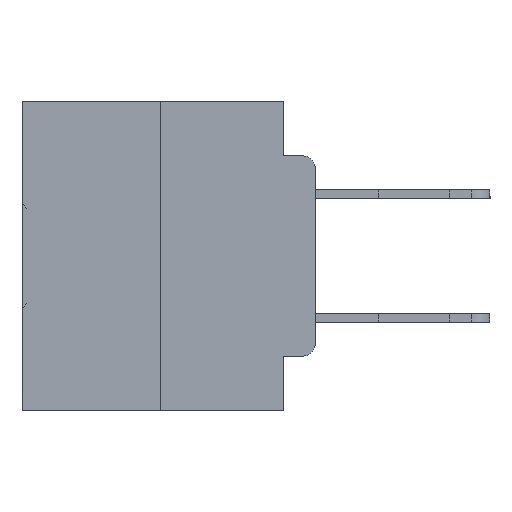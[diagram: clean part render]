
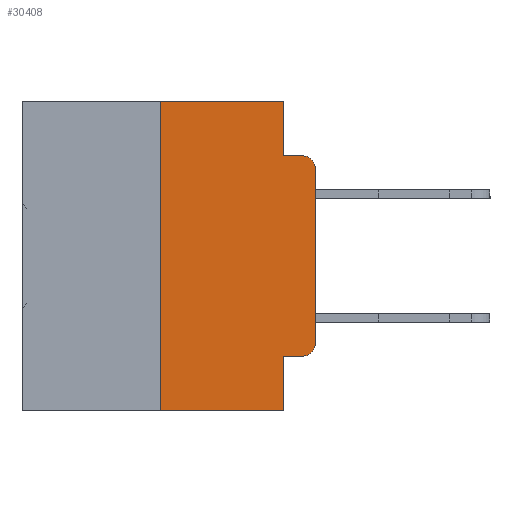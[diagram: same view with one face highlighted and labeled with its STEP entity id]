
A CAD part, left-side view. The second image highlights one B-rep face of the part: STEP entity #30408.
In plain terms, the highlighted planar face has unit normal (-1, 0, 0).
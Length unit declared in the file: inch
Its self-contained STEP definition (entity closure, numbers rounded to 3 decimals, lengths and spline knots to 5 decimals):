
#230 = DIRECTION ( 'NONE',  ( 0., 0., 1. ) ) ;
#309 = CARTESIAN_POINT ( 'NONE',  ( 0., 0.02, -0.4115 ) ) ;
#893 = AXIS2_PLACEMENT_3D ( 'NONE', #1442, #27420, #12068 ) ;
#911 = ORIENTED_EDGE ( 'NONE', *, *, #17243, .F. ) ;
#1036 = VECTOR ( 'NONE', #23882, 39.37008 ) ;
#1442 = CARTESIAN_POINT ( 'NONE',  ( 0., 0.473, 0. ) ) ;
#1462 = DIRECTION ( 'NONE',  ( -1., 0., 0. ) ) ;
#1540 = LINE ( 'NONE', #7301, #21604 ) ;
#2047 = AXIS2_PLACEMENT_3D ( 'NONE', #17199, #1462, #19800 ) ;
#2131 = VECTOR ( 'NONE', #27303, 39.37008 ) ;
#2607 = CARTESIAN_POINT ( 'NONE',  ( 0., 0.051, -0.4115 ) ) ;
#3167 = CARTESIAN_POINT ( 'NONE',  ( 0., 0.051, 0. ) ) ;
#3987 = DIRECTION ( 'NONE',  ( -1., 0., 0. ) ) ;
#4912 = EDGE_CURVE ( 'NONE', #25032, #22070, #17927, .T. ) ;
#5413 = LINE ( 'NONE', #2607, #19292 ) ;
#5738 = DIRECTION ( 'NONE',  ( 0., -1., 0. ) ) ;
#6139 = AXIS2_PLACEMENT_3D ( 'NONE', #19637, #3987, #22230 ) ;
#6345 = ORIENTED_EDGE ( 'NONE', *, *, #9194, .F. ) ;
#6702 = CARTESIAN_POINT ( 'NONE',  ( 0., 0.473, 0. ) ) ;
#6966 = LINE ( 'NONE', #25739, #15532 ) ;
#7089 = EDGE_CURVE ( 'NONE', #31402, #33297, #17375, .T. ) ;
#7301 = CARTESIAN_POINT ( 'NONE',  ( 0., 0.473, -0.5 ) ) ;
#7318 = CARTESIAN_POINT ( 'NONE',  ( 0., 0.051, 0. ) ) ;
#7378 = ORIENTED_EDGE ( 'NONE', *, *, #21119, .T. ) ;
#7640 = FACE_OUTER_BOUND ( 'NONE', #31909, .T. ) ;
#7711 = DIRECTION ( 'NONE',  ( 0., 0., 1. ) ) ;
#7778 = VERTEX_POINT ( 'NONE', #29662 ) ;
#9156 = VERTEX_POINT ( 'NONE', #15133 ) ;
#9183 = LINE ( 'NONE', #6702, #2131 ) ;
#9194 = EDGE_CURVE ( 'NONE', #7778, #32922, #9557, .T. ) ;
#9280 = ORIENTED_EDGE ( 'NONE', *, *, #4912, .F. ) ;
#9343 = EDGE_CURVE ( 'NONE', #25032, #31402, #5413, .T. ) ;
#9557 = LINE ( 'NONE', #23004, #15660 ) ;
#10035 = VECTOR ( 'NONE', #230, 39.37008 ) ;
#11731 = EDGE_CURVE ( 'NONE', #33297, #32806, #6966, .T. ) ;
#12068 = DIRECTION ( 'NONE',  ( 0., 0., -1. ) ) ;
#12513 = DIRECTION ( 'NONE',  ( 0., -1., 0. ) ) ;
#13423 = CARTESIAN_POINT ( 'NONE',  ( 0., 0.25, 0. ) ) ;
#14202 = CARTESIAN_POINT ( 'NONE',  ( 0., 0.02, -0.0885 ) ) ;
#14265 = LINE ( 'NONE', #3167, #1036 ) ;
#15133 = CARTESIAN_POINT ( 'NONE',  ( 0., 0.25, 0. ) ) ;
#15532 = VECTOR ( 'NONE', #7711, 39.37008 ) ;
#15660 = VECTOR ( 'NONE', #12513, 39.37008 ) ;
#16231 = CIRCLE ( 'NONE', #2047, 0.02 ) ;
#16683 = CARTESIAN_POINT ( 'NONE',  ( 0., 0.25, -0.5 ) ) ;
#17199 = CARTESIAN_POINT ( 'NONE',  ( 0., 0.02, -0.1085 ) ) ;
#17243 = EDGE_CURVE ( 'NONE', #9156, #23777, #9183, .T. ) ;
#17375 = CIRCLE ( 'NONE', #6139, 0.02 ) ;
#17927 = LINE ( 'NONE', #21235, #24719 ) ;
#19190 = DIRECTION ( 'NONE',  ( 0., 0., -1. ) ) ;
#19292 = VECTOR ( 'NONE', #5738, 39.37008 ) ;
#19384 = EDGE_CURVE ( 'NONE', #26133, #22070, #1540, .T. ) ;
#19637 = CARTESIAN_POINT ( 'NONE',  ( 0., 0.02, -0.3915 ) ) ;
#19774 = PLANE ( 'NONE',  #893 ) ;
#19800 = DIRECTION ( 'NONE',  ( 0., 0., -1. ) ) ;
#21119 = EDGE_CURVE ( 'NONE', #32806, #32922, #16231, .T. ) ;
#21235 = CARTESIAN_POINT ( 'NONE',  ( 0., 0.051, 0. ) ) ;
#21604 = VECTOR ( 'NONE', #25354, 39.37008 ) ;
#21758 = ORIENTED_EDGE ( 'NONE', *, *, #25485, .F. ) ;
#22036 = CARTESIAN_POINT ( 'NONE',  ( 0., 0.051, -0.4115 ) ) ;
#22070 = VERTEX_POINT ( 'NONE', #28090 ) ;
#22230 = DIRECTION ( 'NONE',  ( 0., 0., -1. ) ) ;
#22249 = ORIENTED_EDGE ( 'NONE', *, *, #19384, .T. ) ;
#23004 = CARTESIAN_POINT ( 'NONE',  ( 0., 0.051, -0.0885 ) ) ;
#23139 = ORIENTED_EDGE ( 'NONE', *, *, #9343, .T. ) ;
#23777 = VERTEX_POINT ( 'NONE', #7318 ) ;
#23882 = DIRECTION ( 'NONE',  ( 0., 0., -1. ) ) ;
#24544 = ORIENTED_EDGE ( 'NONE', *, *, #30736, .F. ) ;
#24719 = VECTOR ( 'NONE', #19190, 39.37008 ) ;
#25032 = VERTEX_POINT ( 'NONE', #22036 ) ;
#25354 = DIRECTION ( 'NONE',  ( 0., -1., 0. ) ) ;
#25485 = EDGE_CURVE ( 'NONE', #23777, #7778, #14265, .T. ) ;
#25739 = CARTESIAN_POINT ( 'NONE',  ( 0., 0., 0. ) ) ;
#26046 = CARTESIAN_POINT ( 'NONE',  ( 0., 0., -0.3915 ) ) ;
#26133 = VERTEX_POINT ( 'NONE', #16683 ) ;
#26235 = ORIENTED_EDGE ( 'NONE', *, *, #7089, .T. ) ;
#27303 = DIRECTION ( 'NONE',  ( 0., -1., 0. ) ) ;
#27420 = DIRECTION ( 'NONE',  ( 1., 0., 0. ) ) ;
#28090 = CARTESIAN_POINT ( 'NONE',  ( 0., 0.051, -0.5 ) ) ;
#29662 = CARTESIAN_POINT ( 'NONE',  ( 0., 0.051, -0.0885 ) ) ;
#30257 = ORIENTED_EDGE ( 'NONE', *, *, #11731, .T. ) ;
#30408 = ADVANCED_FACE ( 'NONE', ( #7640 ), #19774, .F. ) ;
#30481 = LINE ( 'NONE', #13423, #10035 ) ;
#30736 = EDGE_CURVE ( 'NONE', #26133, #9156, #30481, .T. ) ;
#31402 = VERTEX_POINT ( 'NONE', #309 ) ;
#31909 = EDGE_LOOP ( 'NONE', ( #30257, #7378, #6345, #21758, #911, #24544, #22249, #9280, #23139, #26235 ) ) ;
#32029 = CARTESIAN_POINT ( 'NONE',  ( 0., 0., -0.1085 ) ) ;
#32806 = VERTEX_POINT ( 'NONE', #32029 ) ;
#32922 = VERTEX_POINT ( 'NONE', #14202 ) ;
#33297 = VERTEX_POINT ( 'NONE', #26046 ) ;
